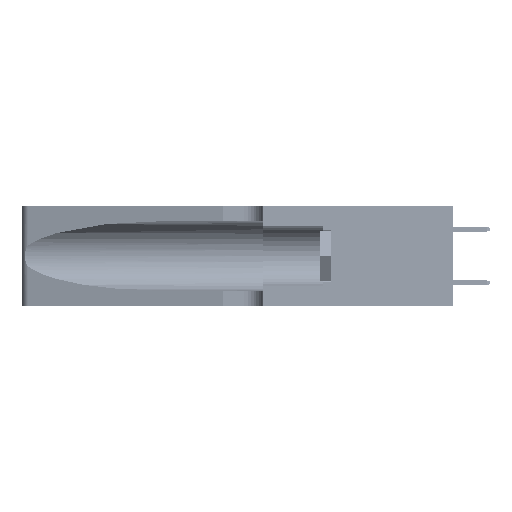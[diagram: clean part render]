
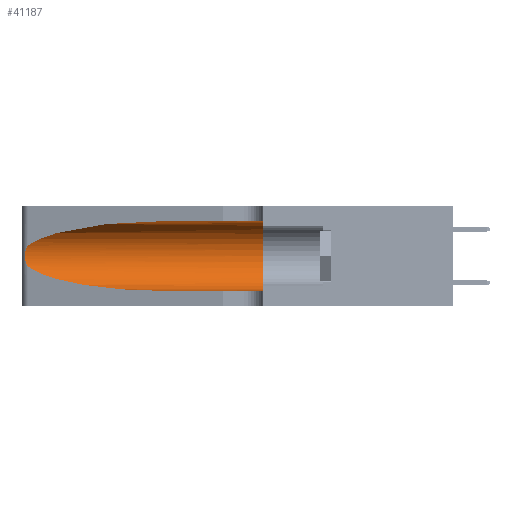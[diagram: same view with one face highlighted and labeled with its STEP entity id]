
A CAD part, left-side view. The second image highlights one B-rep face of the part: STEP entity #41187.
In plain terms, the highlighted cylindrical face has radius 3.308 mm (diameter 6.617 mm), a partial arc.
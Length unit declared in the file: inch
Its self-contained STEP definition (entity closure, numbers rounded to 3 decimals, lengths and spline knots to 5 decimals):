
#934 = VERTEX_POINT ( 'NONE', #31151 ) ;
#1254 = ORIENTED_EDGE ( 'NONE', *, *, #48063, .T. ) ;
#1323 = ORIENTED_EDGE ( 'NONE', *, *, #7969, .T. ) ;
#2517 = CARTESIAN_POINT ( 'NONE',  ( 0.25487, 1.22718, 0.22369 ) ) ;
#2758 = CARTESIAN_POINT ( 'NONE',  ( 0.25555, 1.22994, 0.2215 ) ) ;
#3073 = DIRECTION ( 'NONE',  ( 0., 0., -1. ) ) ;
#3253 = DIRECTION ( 'NONE',  ( 0., -1., 0. ) ) ;
#3513 = CARTESIAN_POINT ( 'NONE',  ( 0.25856, 1.23593, 0.16098 ) ) ;
#6238 = VERTEX_POINT ( 'NONE', #12192 ) ;
#6360 = CARTESIAN_POINT ( 'NONE',  ( 0.25787, 1.23484, 0.2124 ) ) ;
#7253 = EDGE_CURVE ( 'NONE', #12565, #24906, #16353, .T. ) ;
#7406 = CARTESIAN_POINT ( 'NONE',  ( 0.1305, 1.61858, 0.185 ) ) ;
#7969 = EDGE_CURVE ( 'NONE', #30506, #934, #23948, .T. ) ;
#8572 = EDGE_CURVE ( 'NONE', #9461, #934, #48336, .T. ) ;
#9461 = VERTEX_POINT ( 'NONE', #36236 ) ;
#11172 = CARTESIAN_POINT ( 'NONE',  ( 0.25789, 1.23486, 0.15765 ) ) ;
#11340 = ORIENTED_EDGE ( 'NONE', *, *, #17229, .F. ) ;
#12192 = CARTESIAN_POINT ( 'NONE',  ( 0.25487, 1.22718, 0.14631 ) ) ;
#12565 = VERTEX_POINT ( 'NONE', #29195 ) ;
#13193 = DIRECTION ( 'NONE',  ( 0., 0., 1. ) ) ;
#13352 = ORIENTED_EDGE ( 'NONE', *, *, #7253, .T. ) ;
#15534 = DIRECTION ( 'NONE',  ( 0., -1., 0. ) ) ;
#16353 =( BOUNDED_CURVE ( )  B_SPLINE_CURVE ( 3, ( #16903, #28602, #43904, #28106 ),
 .UNSPECIFIED., .F., .T. ) 
 B_SPLINE_CURVE_WITH_KNOTS ( ( 4, 4 ),
 ( 1.5708, 2.84003 ),
 .UNSPECIFIED. ) 
 CURVE ( )  GEOMETRIC_REPRESENTATION_ITEM ( )  RATIONAL_B_SPLINE_CURVE ( ( 1., 0.87, 0.87, 1. ) ) 
 REPRESENTATION_ITEM ( '' )  );
#16568 = CARTESIAN_POINT ( 'NONE',  ( 0.1305, 1.61858, 0.05475 ) ) ;
#16903 = CARTESIAN_POINT ( 'NONE',  ( 0.1305, 0.72297, 0.31525 ) ) ;
#16997 = CARTESIAN_POINT ( 'NONE',  ( 0.2373, 1.15595, 0.08982 ) ) ;
#17229 = EDGE_CURVE ( 'NONE', #12565, #9461, #31019, .T. ) ;
#18792 = CARTESIAN_POINT ( 'NONE',  ( 0.25854, 1.2359, 0.20912 ) ) ;
#19105 = FACE_OUTER_BOUND ( 'NONE', #25356, .T. ) ;
#19621 = DIRECTION ( 'NONE',  ( 0., -1., 0. ) ) ;
#21528 = VECTOR ( 'NONE', #19621, 39.37008 ) ;
#21833 = CARTESIAN_POINT ( 'NONE',  ( 0.1305, 0.35, 0.185 ) ) ;
#23948 = LINE ( 'NONE', #16568, #21528 ) ;
#24250 = CARTESIAN_POINT ( 'NONE',  ( 0.1305, 0.72297, 0.05475 ) ) ;
#24906 = VERTEX_POINT ( 'NONE', #27695 ) ;
#25356 = EDGE_LOOP ( 'NONE', ( #13352, #47747, #1254, #1323, #43045, #11340 ) ) ;
#25702 = CARTESIAN_POINT ( 'NONE',  ( 0.26075, 1.23896, 0.19203 ) ) ;
#27695 = CARTESIAN_POINT ( 'NONE',  ( 0.25487, 1.22718, 0.22369 ) ) ;
#28106 = CARTESIAN_POINT ( 'NONE',  ( 0.25487, 1.22718, 0.22369 ) ) ;
#28602 = CARTESIAN_POINT ( 'NONE',  ( 0.18966, 0.96281, 0.31525 ) ) ;
#28949 = CARTESIAN_POINT ( 'NONE',  ( 0.18966, 0.96281, 0.05475 ) ) ;
#29195 = CARTESIAN_POINT ( 'NONE',  ( 0.1305, 0.72297, 0.31525 ) ) ;
#29522 = CARTESIAN_POINT ( 'NONE',  ( 0.25487, 1.22718, 0.14631 ) ) ;
#29781 = CARTESIAN_POINT ( 'NONE',  ( 0.25639, 1.23184, 0.21858 ) ) ;
#30506 = VERTEX_POINT ( 'NONE', #24250 ) ;
#31019 = LINE ( 'NONE', #34586, #37396 ) ;
#31151 = CARTESIAN_POINT ( 'NONE',  ( 0.1305, 0.35, 0.05475 ) ) ;
#34037 = EDGE_CURVE ( 'NONE', #24906, #6238, #47840, .T. ) ;
#34586 = CARTESIAN_POINT ( 'NONE',  ( 0.1305, 1.61858, 0.31525 ) ) ;
#35233 =( BOUNDED_CURVE ( )  B_SPLINE_CURVE ( 3, ( #48319, #16997, #28949, #40405 ),
 .UNSPECIFIED., .F., .T. ) 
 B_SPLINE_CURVE_WITH_KNOTS ( ( 4, 4 ),
 ( 3.44316, 4.71239 ),
 .UNSPECIFIED. ) 
 CURVE ( )  GEOMETRIC_REPRESENTATION_ITEM ( )  RATIONAL_B_SPLINE_CURVE ( ( 1., 0.87, 0.87, 1. ) ) 
 REPRESENTATION_ITEM ( '' )  );
#36236 = CARTESIAN_POINT ( 'NONE',  ( 0.1305, 0.35, 0.31525 ) ) ;
#37396 = VECTOR ( 'NONE', #3253, 39.37008 ) ;
#37641 = CARTESIAN_POINT ( 'NONE',  ( 0.25555, 1.22993, 0.14849 ) ) ;
#37948 = CYLINDRICAL_SURFACE ( 'NONE', #38669, 0.13025 ) ;
#38400 = CARTESIAN_POINT ( 'NONE',  ( 0.26017, 1.23833, 0.17102 ) ) ;
#38669 = AXIS2_PLACEMENT_3D ( 'NONE', #7406, #15534, #3073 ) ;
#40405 = CARTESIAN_POINT ( 'NONE',  ( 0.1305, 0.72297, 0.05475 ) ) ;
#41180 = DIRECTION ( 'NONE',  ( 0., 1., 0. ) ) ;
#41187 = ADVANCED_FACE ( 'NONE', ( #19105 ), #37948, .F. ) ;
#43045 = ORIENTED_EDGE ( 'NONE', *, *, #8572, .F. ) ;
#43904 = CARTESIAN_POINT ( 'NONE',  ( 0.2373, 1.15595, 0.28018 ) ) ;
#44247 = AXIS2_PLACEMENT_3D ( 'NONE', #21833, #41180, #13193 ) ;
#45310 = CARTESIAN_POINT ( 'NONE',  ( 0.25639, 1.23186, 0.15144 ) ) ;
#45566 = CARTESIAN_POINT ( 'NONE',  ( 0.26075, 1.23896, 0.178 ) ) ;
#46070 = CARTESIAN_POINT ( 'NONE',  ( 0.26018, 1.23835, 0.19895 ) ) ;
#47747 = ORIENTED_EDGE ( 'NONE', *, *, #34037, .T. ) ;
#47840 = B_SPLINE_CURVE_WITH_KNOTS ( 'NONE', 3,
 ( #2517, #2758, #29781, #6360, #18792, #46070, #25702, #45566, #38400, #3513, #11172, #45310, #37641, #29522 ),
 .UNSPECIFIED., .F., .F.,
 ( 4, 2, 2, 2, 2, 2, 4 ),
 ( 0., 0.00027, 0.00053, 0.00107, 0.0016, 0.00187, 0.00214 ),
 .UNSPECIFIED. ) ;
#48063 = EDGE_CURVE ( 'NONE', #6238, #30506, #35233, .T. ) ;
#48319 = CARTESIAN_POINT ( 'NONE',  ( 0.25487, 1.22718, 0.14631 ) ) ;
#48336 = CIRCLE ( 'NONE', #44247, 0.13025 ) ;
